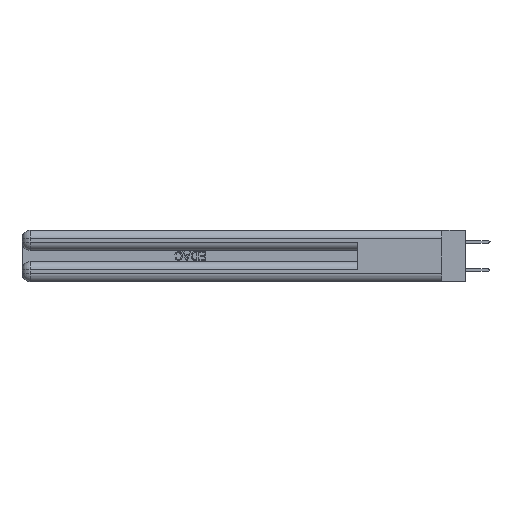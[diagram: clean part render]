
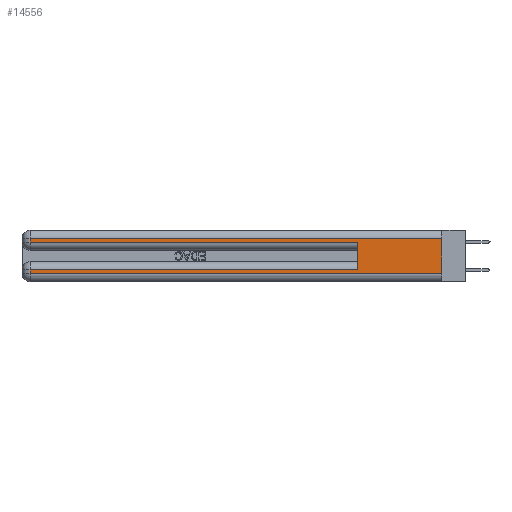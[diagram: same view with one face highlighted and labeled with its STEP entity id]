
A CAD part, left-side view. The second image highlights one B-rep face of the part: STEP entity #14556.
In plain terms, the highlighted planar face has unit normal (-1, 0, 0).
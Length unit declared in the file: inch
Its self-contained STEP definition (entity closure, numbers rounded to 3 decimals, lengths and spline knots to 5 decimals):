
#741 = ORIENTED_EDGE ( 'NONE', *, *, #2588, .T. ) ;
#953 = VERTEX_POINT ( 'NONE', #31078 ) ;
#2588 = EDGE_CURVE ( 'NONE', #8818, #953, #35400, .T. ) ;
#3496 = EDGE_CURVE ( 'NONE', #41712, #34991, #19811, .T. ) ;
#3529 = DIRECTION ( 'NONE',  ( 0., -1., 0. ) ) ;
#4209 = LINE ( 'NONE', #15095, #13257 ) ;
#4846 = CARTESIAN_POINT ( 'NONE',  ( 0., 2.94, 0.37 ) ) ;
#5332 = LINE ( 'NONE', #36162, #37948 ) ;
#6783 = VECTOR ( 'NONE', #17005, 39.37008 ) ;
#7893 = DIRECTION ( 'NONE',  ( 0., 0., -1. ) ) ;
#8578 = ORIENTED_EDGE ( 'NONE', *, *, #20626, .F. ) ;
#8818 = VERTEX_POINT ( 'NONE', #32694 ) ;
#9165 = CARTESIAN_POINT ( 'NONE',  ( 0., 0.6, 0.085 ) ) ;
#9425 = EDGE_CURVE ( 'NONE', #14381, #8818, #4209, .T. ) ;
#10587 = ORIENTED_EDGE ( 'NONE', *, *, #9425, .T. ) ;
#11124 = CARTESIAN_POINT ( 'NONE',  ( 0., 2.94, 0.285 ) ) ;
#12202 = CARTESIAN_POINT ( 'NONE',  ( 0., 0., 0.31 ) ) ;
#13019 = VERTEX_POINT ( 'NONE', #14455 ) ;
#13257 = VECTOR ( 'NONE', #7893, 39.37008 ) ;
#14265 = CARTESIAN_POINT ( 'NONE',  ( 0., 2.94, 0.085 ) ) ;
#14381 = VERTEX_POINT ( 'NONE', #14265 ) ;
#14455 = CARTESIAN_POINT ( 'NONE',  ( 0., 0., 0.31 ) ) ;
#14556 = ADVANCED_FACE ( 'NONE', ( #28649 ), #38701, .F. ) ;
#14557 = DIRECTION ( 'NONE',  ( 0., 0., 1. ) ) ;
#15095 = CARTESIAN_POINT ( 'NONE',  ( 0., 2.94, 0.37 ) ) ;
#15727 = DIRECTION ( 'NONE',  ( 0., 1., 0. ) ) ;
#15853 = VERTEX_POINT ( 'NONE', #36051 ) ;
#16194 = VECTOR ( 'NONE', #3529, 39.37008 ) ;
#16235 = EDGE_CURVE ( 'NONE', #17124, #34991, #39198, .T. ) ;
#17005 = DIRECTION ( 'NONE',  ( 0., 0., -1. ) ) ;
#17124 = VERTEX_POINT ( 'NONE', #9165 ) ;
#17648 = CARTESIAN_POINT ( 'NONE',  ( 0., 0.6, 0.145 ) ) ;
#18231 = CARTESIAN_POINT ( 'NONE',  ( 0., 0., 0.37 ) ) ;
#18286 = EDGE_LOOP ( 'NONE', ( #8578, #30276, #19247, #30985, #41312, #33492, #10587, #741 ) ) ;
#19247 = ORIENTED_EDGE ( 'NONE', *, *, #35256, .T. ) ;
#19811 = LINE ( 'NONE', #31123, #24615 ) ;
#20626 = EDGE_CURVE ( 'NONE', #13019, #953, #26532, .T. ) ;
#23508 = VECTOR ( 'NONE', #29017, 39.37008 ) ;
#23848 = AXIS2_PLACEMENT_3D ( 'NONE', #18231, #42150, #31990 ) ;
#23964 = CARTESIAN_POINT ( 'NONE',  ( 0., 0., 0.06 ) ) ;
#24615 = VECTOR ( 'NONE', #34393, 39.37008 ) ;
#26532 = LINE ( 'NONE', #30599, #6783 ) ;
#28649 = FACE_OUTER_BOUND ( 'NONE', #18286, .T. ) ;
#29017 = DIRECTION ( 'NONE',  ( 0., 0., -1. ) ) ;
#29585 = LINE ( 'NONE', #12202, #44024 ) ;
#30276 = ORIENTED_EDGE ( 'NONE', *, *, #32777, .T. ) ;
#30599 = CARTESIAN_POINT ( 'NONE',  ( 0., 0., 0.37 ) ) ;
#30985 = ORIENTED_EDGE ( 'NONE', *, *, #3496, .T. ) ;
#31078 = CARTESIAN_POINT ( 'NONE',  ( 0., 0., 0.06 ) ) ;
#31123 = CARTESIAN_POINT ( 'NONE',  ( 0., 0., 0.285 ) ) ;
#31990 = DIRECTION ( 'NONE',  ( 0., 0., -1. ) ) ;
#32694 = CARTESIAN_POINT ( 'NONE',  ( 0., 2.94, 0.06 ) ) ;
#32777 = EDGE_CURVE ( 'NONE', #13019, #15853, #29585, .T. ) ;
#33492 = ORIENTED_EDGE ( 'NONE', *, *, #35320, .T. ) ;
#34393 = DIRECTION ( 'NONE',  ( 0., -1., 0. ) ) ;
#34991 = VERTEX_POINT ( 'NONE', #40861 ) ;
#35256 = EDGE_CURVE ( 'NONE', #15853, #41712, #43810, .T. ) ;
#35320 = EDGE_CURVE ( 'NONE', #17124, #14381, #5332, .T. ) ;
#35400 = LINE ( 'NONE', #23964, #16194 ) ;
#35766 = DIRECTION ( 'NONE',  ( 0., 1., 0. ) ) ;
#36051 = CARTESIAN_POINT ( 'NONE',  ( 0., 2.94, 0.31 ) ) ;
#36162 = CARTESIAN_POINT ( 'NONE',  ( 0., 0., 0.085 ) ) ;
#37948 = VECTOR ( 'NONE', #15727, 39.37008 ) ;
#38701 = PLANE ( 'NONE',  #23848 ) ;
#39198 = LINE ( 'NONE', #17648, #39704 ) ;
#39704 = VECTOR ( 'NONE', #14557, 39.37008 ) ;
#40861 = CARTESIAN_POINT ( 'NONE',  ( 0., 0.6, 0.285 ) ) ;
#41312 = ORIENTED_EDGE ( 'NONE', *, *, #16235, .F. ) ;
#41712 = VERTEX_POINT ( 'NONE', #11124 ) ;
#42150 = DIRECTION ( 'NONE',  ( 1., 0., 0. ) ) ;
#43810 = LINE ( 'NONE', #4846, #23508 ) ;
#44024 = VECTOR ( 'NONE', #35766, 39.37008 ) ;
